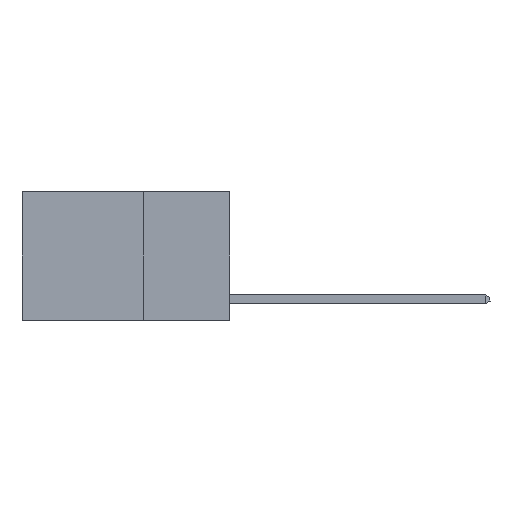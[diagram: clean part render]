
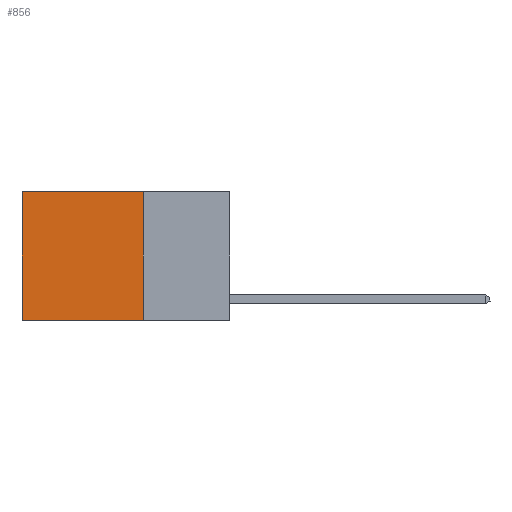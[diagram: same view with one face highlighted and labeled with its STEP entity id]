
A CAD part, left-side view. The second image highlights one B-rep face of the part: STEP entity #856.
In plain terms, the highlighted planar face has unit normal (-1, 0, 0).
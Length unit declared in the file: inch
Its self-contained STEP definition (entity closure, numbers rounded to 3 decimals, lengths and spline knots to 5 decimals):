
#478 = ORIENTED_EDGE ( 'NONE', *, *, #10295, .T. ) ;
#856 = ADVANCED_FACE ( 'NONE', ( #7138 ), #9683, .F. ) ;
#865 = VERTEX_POINT ( 'NONE', #3886 ) ;
#1406 = CARTESIAN_POINT ( 'NONE',  ( 0.2625, 0.25, 0. ) ) ;
#2073 = DIRECTION ( 'NONE',  ( 0., 0., -1. ) ) ;
#2826 = VERTEX_POINT ( 'NONE', #21585 ) ;
#3734 = DIRECTION ( 'NONE',  ( 0., 1., 0. ) ) ;
#3886 = CARTESIAN_POINT ( 'NONE',  ( 0.2625, 0.6, 0. ) ) ;
#4081 = EDGE_LOOP ( 'NONE', ( #21989, #14229, #22661, #478 ) ) ;
#4158 = VECTOR ( 'NONE', #9999, 39.37008 ) ;
#4483 = CARTESIAN_POINT ( 'NONE',  ( 0.2625, 0.6, -0.37 ) ) ;
#4766 = VECTOR ( 'NONE', #3734, 39.37008 ) ;
#5058 = LINE ( 'NONE', #1406, #4766 ) ;
#6966 = EDGE_CURVE ( 'NONE', #2826, #23819, #16054, .T. ) ;
#7084 = LINE ( 'NONE', #9554, #22227 ) ;
#7138 = FACE_OUTER_BOUND ( 'NONE', #4081, .T. ) ;
#9554 = CARTESIAN_POINT ( 'NONE',  ( 0.2625, 0.6, 0. ) ) ;
#9613 = DIRECTION ( 'NONE',  ( 0., 1., 0. ) ) ;
#9683 = PLANE ( 'NONE',  #20432 ) ;
#9999 = DIRECTION ( 'NONE',  ( 0., 0., -1. ) ) ;
#10295 = EDGE_CURVE ( 'NONE', #2826, #865, #5058, .T. ) ;
#12239 = LINE ( 'NONE', #15085, #23847 ) ;
#14229 = ORIENTED_EDGE ( 'NONE', *, *, #19271, .F. ) ;
#15031 = CARTESIAN_POINT ( 'NONE',  ( 0.2625, 0.25, -0.37 ) ) ;
#15085 = CARTESIAN_POINT ( 'NONE',  ( 0.2625, 0.25, -0.37 ) ) ;
#15647 = CARTESIAN_POINT ( 'NONE',  ( 0.2625, 0.25, 0. ) ) ;
#16054 = LINE ( 'NONE', #15647, #4158 ) ;
#17232 = CARTESIAN_POINT ( 'NONE',  ( 0.2625, 0.25, 0. ) ) ;
#17471 = VERTEX_POINT ( 'NONE', #4483 ) ;
#19271 = EDGE_CURVE ( 'NONE', #23819, #17471, #12239, .T. ) ;
#20432 = AXIS2_PLACEMENT_3D ( 'NONE', #17232, #23057, #21004 ) ;
#21004 = DIRECTION ( 'NONE',  ( 0., 0., -1. ) ) ;
#21029 = EDGE_CURVE ( 'NONE', #865, #17471, #7084, .T. ) ;
#21585 = CARTESIAN_POINT ( 'NONE',  ( 0.2625, 0.25, 0. ) ) ;
#21989 = ORIENTED_EDGE ( 'NONE', *, *, #21029, .T. ) ;
#22227 = VECTOR ( 'NONE', #2073, 39.37008 ) ;
#22661 = ORIENTED_EDGE ( 'NONE', *, *, #6966, .F. ) ;
#23057 = DIRECTION ( 'NONE',  ( 1., 0., 0. ) ) ;
#23819 = VERTEX_POINT ( 'NONE', #15031 ) ;
#23847 = VECTOR ( 'NONE', #9613, 39.37008 ) ;
